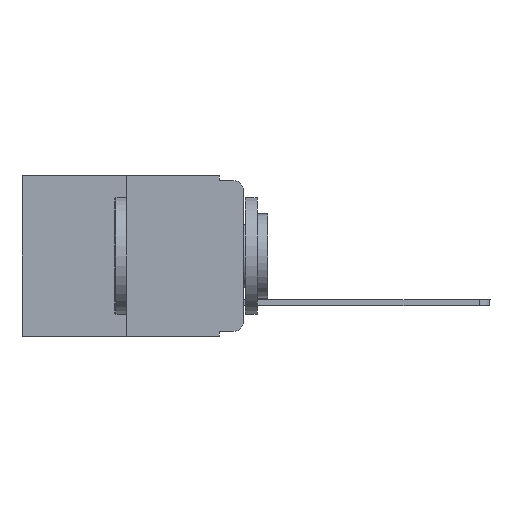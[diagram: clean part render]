
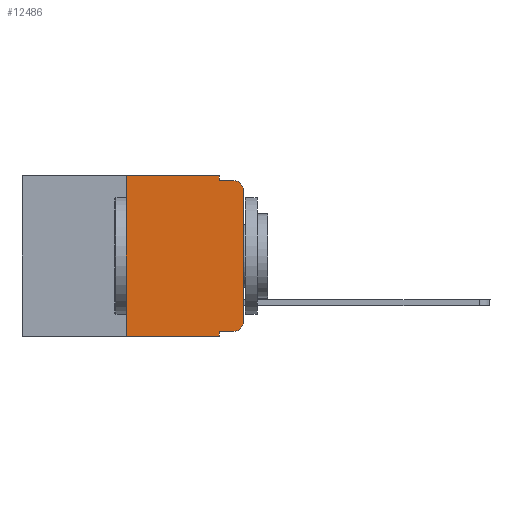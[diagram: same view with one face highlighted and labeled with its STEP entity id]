
A CAD part, left-side view. The second image highlights one B-rep face of the part: STEP entity #12486.
In plain terms, the highlighted planar face has unit normal (-1, 0, 0).
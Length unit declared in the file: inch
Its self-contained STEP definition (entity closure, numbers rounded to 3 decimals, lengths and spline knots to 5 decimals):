
#500 = ORIENTED_EDGE ( 'NONE', *, *, #2050, .F. ) ;
#609 = VERTEX_POINT ( 'NONE', #1308 ) ;
#733 = LINE ( 'NONE', #13511, #9063 ) ;
#933 = LINE ( 'NONE', #3929, #3995 ) ;
#1124 = ORIENTED_EDGE ( 'NONE', *, *, #3026, .T. ) ;
#1156 = ORIENTED_EDGE ( 'NONE', *, *, #9397, .T. ) ;
#1308 = CARTESIAN_POINT ( 'NONE',  ( 0., 0.02, -0.01 ) ) ;
#1338 = DIRECTION ( 'NONE',  ( 0., 0., -1. ) ) ;
#1511 = CARTESIAN_POINT ( 'NONE',  ( 0., 0.051, -0.01 ) ) ;
#1514 = LINE ( 'NONE', #10129, #12412 ) ;
#1543 = CARTESIAN_POINT ( 'NONE',  ( 0., 0.051, -0.333 ) ) ;
#1601 = EDGE_CURVE ( 'NONE', #9544, #609, #733, .T. ) ;
#1605 = DIRECTION ( 'NONE',  ( -1., 0., 0. ) ) ;
#1833 = DIRECTION ( 'NONE',  ( 0., 0., -1. ) ) ;
#2050 = EDGE_CURVE ( 'NONE', #3099, #9654, #12687, .T. ) ;
#2418 = VERTEX_POINT ( 'NONE', #11846 ) ;
#3026 = EDGE_CURVE ( 'NONE', #7436, #609, #10249, .T. ) ;
#3099 = VERTEX_POINT ( 'NONE', #12627 ) ;
#3230 = DIRECTION ( 'NONE',  ( 0., 0., -1. ) ) ;
#3308 = VECTOR ( 'NONE', #4884, 39.37008 ) ;
#3561 = EDGE_CURVE ( 'NONE', #3099, #12338, #1514, .T. ) ;
#3672 = VECTOR ( 'NONE', #11729, 39.37008 ) ;
#3763 = EDGE_CURVE ( 'NONE', #9755, #2418, #9475, .T. ) ;
#3785 = ORIENTED_EDGE ( 'NONE', *, *, #3561, .T. ) ;
#3929 = CARTESIAN_POINT ( 'NONE',  ( 0., 0.473, 0. ) ) ;
#3995 = VECTOR ( 'NONE', #14372, 39.37008 ) ;
#4216 = ORIENTED_EDGE ( 'NONE', *, *, #3763, .T. ) ;
#4700 = EDGE_CURVE ( 'NONE', #9654, #8306, #933, .T. ) ;
#4751 = EDGE_CURVE ( 'NONE', #2418, #6960, #10541, .T. ) ;
#4884 = DIRECTION ( 'NONE',  ( 0., 0., 1. ) ) ;
#5132 = DIRECTION ( 'NONE',  ( 0., 0., 1. ) ) ;
#5419 = PLANE ( 'NONE',  #11977 ) ;
#5503 = DIRECTION ( 'NONE',  ( 0., -1., 0. ) ) ;
#5946 = EDGE_LOOP ( 'NONE', ( #1156, #1124, #8962, #6275, #7168, #500, #3785, #13405, #4216, #6788 ) ) ;
#6166 = CARTESIAN_POINT ( 'NONE',  ( 0., 0., -0.313 ) ) ;
#6273 = CARTESIAN_POINT ( 'NONE',  ( 0., 0.02, -0.313 ) ) ;
#6275 = ORIENTED_EDGE ( 'NONE', *, *, #10418, .F. ) ;
#6512 = VECTOR ( 'NONE', #5132, 39.37008 ) ;
#6760 = EDGE_CURVE ( 'NONE', #9755, #12338, #10496, .T. ) ;
#6788 = ORIENTED_EDGE ( 'NONE', *, *, #4751, .T. ) ;
#6960 = VERTEX_POINT ( 'NONE', #6166 ) ;
#7153 = CARTESIAN_POINT ( 'NONE',  ( 0., 0.051, 0. ) ) ;
#7168 = ORIENTED_EDGE ( 'NONE', *, *, #4700, .F. ) ;
#7436 = VERTEX_POINT ( 'NONE', #11722 ) ;
#7848 = DIRECTION ( 'NONE',  ( 0., -1., 0. ) ) ;
#7921 = AXIS2_PLACEMENT_3D ( 'NONE', #6273, #1605, #14404 ) ;
#7932 = CARTESIAN_POINT ( 'NONE',  ( 0., 0.051, -0.333 ) ) ;
#8306 = VERTEX_POINT ( 'NONE', #10857 ) ;
#8602 = CARTESIAN_POINT ( 'NONE',  ( 0., 0.25, 0. ) ) ;
#8684 = VECTOR ( 'NONE', #10630, 39.37008 ) ;
#8962 = ORIENTED_EDGE ( 'NONE', *, *, #1601, .F. ) ;
#9063 = VECTOR ( 'NONE', #5503, 39.37008 ) ;
#9397 = EDGE_CURVE ( 'NONE', #6960, #7436, #13271, .T. ) ;
#9475 = LINE ( 'NONE', #1543, #3672 ) ;
#9544 = VERTEX_POINT ( 'NONE', #1511 ) ;
#9645 = AXIS2_PLACEMENT_3D ( 'NONE', #11893, #9823, #3230 ) ;
#9654 = VERTEX_POINT ( 'NONE', #12265 ) ;
#9755 = VERTEX_POINT ( 'NONE', #7932 ) ;
#9823 = DIRECTION ( 'NONE',  ( -1., 0., 0. ) ) ;
#10129 = CARTESIAN_POINT ( 'NONE',  ( 0., 0.473, -0.343 ) ) ;
#10249 = CIRCLE ( 'NONE', #9645, 0.02 ) ;
#10418 = EDGE_CURVE ( 'NONE', #8306, #9544, #10698, .T. ) ;
#10496 = LINE ( 'NONE', #13962, #8684 ) ;
#10541 = CIRCLE ( 'NONE', #7921, 0.02 ) ;
#10630 = DIRECTION ( 'NONE',  ( 0., 0., -1. ) ) ;
#10698 = LINE ( 'NONE', #7153, #11788 ) ;
#10857 = CARTESIAN_POINT ( 'NONE',  ( 0., 0.051, 0. ) ) ;
#11722 = CARTESIAN_POINT ( 'NONE',  ( 0., 0., -0.03 ) ) ;
#11729 = DIRECTION ( 'NONE',  ( 0., -1., 0. ) ) ;
#11788 = VECTOR ( 'NONE', #1338, 39.37008 ) ;
#11846 = CARTESIAN_POINT ( 'NONE',  ( 0., 0.02, -0.333 ) ) ;
#11893 = CARTESIAN_POINT ( 'NONE',  ( 0., 0.02, -0.03 ) ) ;
#11977 = AXIS2_PLACEMENT_3D ( 'NONE', #14480, #14538, #1833 ) ;
#12265 = CARTESIAN_POINT ( 'NONE',  ( 0., 0.25, 0. ) ) ;
#12338 = VERTEX_POINT ( 'NONE', #13230 ) ;
#12412 = VECTOR ( 'NONE', #7848, 39.37008 ) ;
#12486 = ADVANCED_FACE ( 'NONE', ( #14825 ), #5419, .F. ) ;
#12627 = CARTESIAN_POINT ( 'NONE',  ( 0., 0.25, -0.343 ) ) ;
#12687 = LINE ( 'NONE', #8602, #6512 ) ;
#13230 = CARTESIAN_POINT ( 'NONE',  ( 0., 0.051, -0.343 ) ) ;
#13271 = LINE ( 'NONE', #14013, #3308 ) ;
#13405 = ORIENTED_EDGE ( 'NONE', *, *, #6760, .F. ) ;
#13511 = CARTESIAN_POINT ( 'NONE',  ( 0., 0.051, -0.01 ) ) ;
#13962 = CARTESIAN_POINT ( 'NONE',  ( 0., 0.051, 0. ) ) ;
#14013 = CARTESIAN_POINT ( 'NONE',  ( 0., 0., 0. ) ) ;
#14372 = DIRECTION ( 'NONE',  ( 0., -1., 0. ) ) ;
#14404 = DIRECTION ( 'NONE',  ( 0., 0., -1. ) ) ;
#14480 = CARTESIAN_POINT ( 'NONE',  ( 0., 0.473, 0. ) ) ;
#14538 = DIRECTION ( 'NONE',  ( 1., 0., 0. ) ) ;
#14825 = FACE_OUTER_BOUND ( 'NONE', #5946, .T. ) ;
